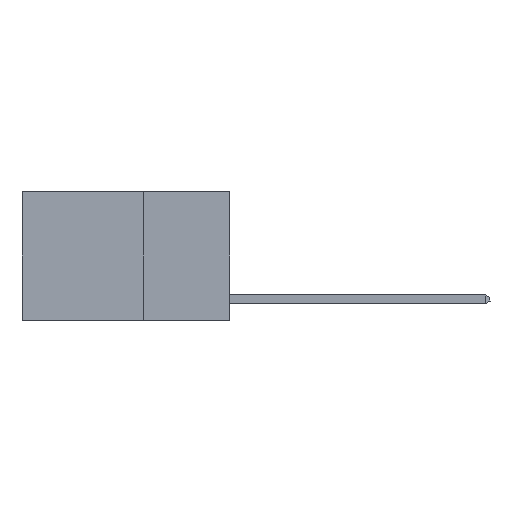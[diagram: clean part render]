
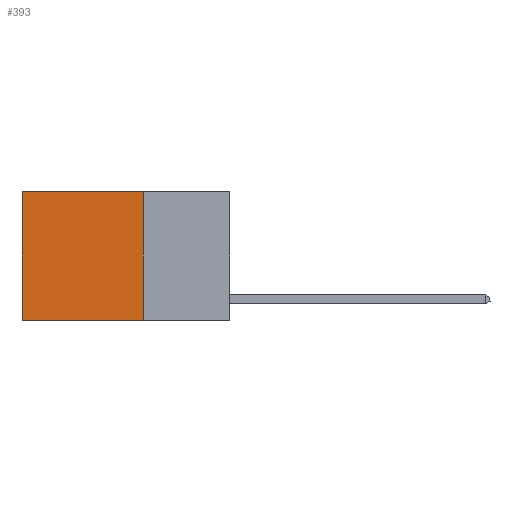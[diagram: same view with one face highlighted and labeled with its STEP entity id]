
A CAD part, left-side view. The second image highlights one B-rep face of the part: STEP entity #393.
In plain terms, the highlighted planar face has unit normal (-1, 0, 0).
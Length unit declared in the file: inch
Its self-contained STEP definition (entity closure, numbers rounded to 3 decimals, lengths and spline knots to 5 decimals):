
#62 = VECTOR ( 'NONE', #8185, 39.37008 ) ;
#393 = ADVANCED_FACE ( 'NONE', ( #12054 ), #2641, .F. ) ;
#822 = ORIENTED_EDGE ( 'NONE', *, *, #6152, .T. ) ;
#844 = ORIENTED_EDGE ( 'NONE', *, *, #10452, .T. ) ;
#1584 = LINE ( 'NONE', #3804, #3651 ) ;
#2537 = VERTEX_POINT ( 'NONE', #9768 ) ;
#2624 = VERTEX_POINT ( 'NONE', #9944 ) ;
#2641 = PLANE ( 'NONE',  #4034 ) ;
#3630 = CARTESIAN_POINT ( 'NONE',  ( 0.2625, 0.25, 0. ) ) ;
#3651 = VECTOR ( 'NONE', #11570, 39.37008 ) ;
#3804 = CARTESIAN_POINT ( 'NONE',  ( 0.2625, 0.25, -0.37 ) ) ;
#4034 = AXIS2_PLACEMENT_3D ( 'NONE', #8157, #4847, #6863 ) ;
#4213 = LINE ( 'NONE', #12597, #6523 ) ;
#4313 = CARTESIAN_POINT ( 'NONE',  ( 0.2625, 0.6, 0. ) ) ;
#4483 = EDGE_CURVE ( 'NONE', #7598, #9758, #10334, .T. ) ;
#4659 = DIRECTION ( 'NONE',  ( 0., 0., -1. ) ) ;
#4847 = DIRECTION ( 'NONE',  ( 1., 0., 0. ) ) ;
#5730 = CARTESIAN_POINT ( 'NONE',  ( 0.2625, 0.25, -0.37 ) ) ;
#6152 = EDGE_CURVE ( 'NONE', #2537, #2624, #8001, .T. ) ;
#6523 = VECTOR ( 'NONE', #11667, 39.37008 ) ;
#6758 = EDGE_CURVE ( 'NONE', #9758, #2624, #1584, .T. ) ;
#6863 = DIRECTION ( 'NONE',  ( 0., 0., -1. ) ) ;
#7221 = CARTESIAN_POINT ( 'NONE',  ( 0.2625, 0.25, 0. ) ) ;
#7598 = VERTEX_POINT ( 'NONE', #7221 ) ;
#7718 = VECTOR ( 'NONE', #4659, 39.37008 ) ;
#8001 = LINE ( 'NONE', #4313, #62 ) ;
#8157 = CARTESIAN_POINT ( 'NONE',  ( 0.2625, 0.25, 0. ) ) ;
#8185 = DIRECTION ( 'NONE',  ( 0., 0., -1. ) ) ;
#8280 = ORIENTED_EDGE ( 'NONE', *, *, #4483, .F. ) ;
#8999 = ORIENTED_EDGE ( 'NONE', *, *, #6758, .F. ) ;
#9758 = VERTEX_POINT ( 'NONE', #5730 ) ;
#9768 = CARTESIAN_POINT ( 'NONE',  ( 0.2625, 0.6, 0. ) ) ;
#9944 = CARTESIAN_POINT ( 'NONE',  ( 0.2625, 0.6, -0.37 ) ) ;
#10334 = LINE ( 'NONE', #3630, #7718 ) ;
#10452 = EDGE_CURVE ( 'NONE', #7598, #2537, #4213, .T. ) ;
#11427 = EDGE_LOOP ( 'NONE', ( #822, #8999, #8280, #844 ) ) ;
#11570 = DIRECTION ( 'NONE',  ( 0., 1., 0. ) ) ;
#11667 = DIRECTION ( 'NONE',  ( 0., 1., 0. ) ) ;
#12054 = FACE_OUTER_BOUND ( 'NONE', #11427, .T. ) ;
#12597 = CARTESIAN_POINT ( 'NONE',  ( 0.2625, 0.25, 0. ) ) ;
